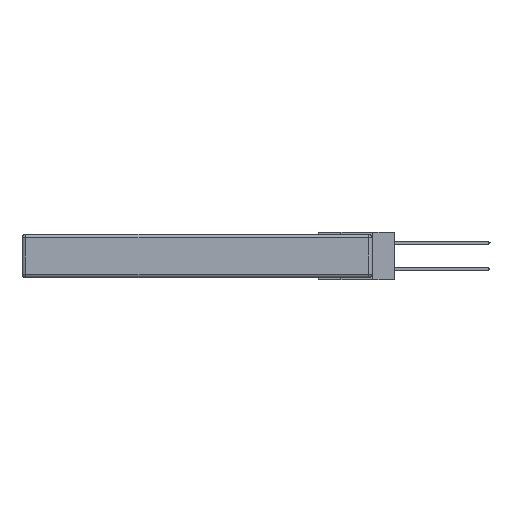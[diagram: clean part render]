
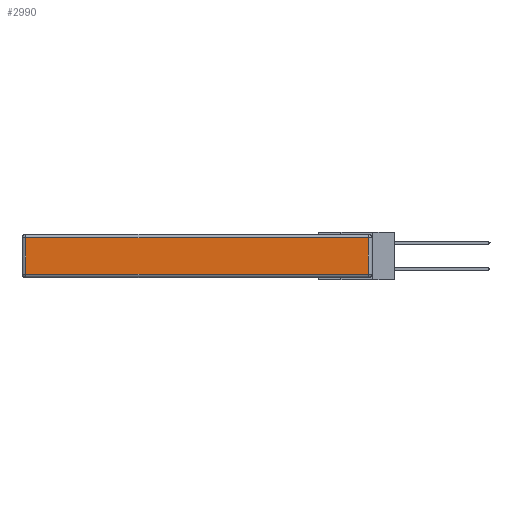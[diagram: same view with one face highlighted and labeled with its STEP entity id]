
A CAD part, left-side view. The second image highlights one B-rep face of the part: STEP entity #2990.
In plain terms, the highlighted planar face has unit normal (-1, 0, 0).
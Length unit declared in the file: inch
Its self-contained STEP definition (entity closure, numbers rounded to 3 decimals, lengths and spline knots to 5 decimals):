
#591 = DIRECTION ( 'NONE',  ( -1., 0., 0. ) ) ;
#1681 = DIRECTION ( 'NONE',  ( 0., -1., 0. ) ) ;
#1724 = CARTESIAN_POINT ( 'NONE',  ( 0., 2.72, -0.03 ) ) ;
#2984 = ORIENTED_EDGE ( 'NONE', *, *, #9275, .T. ) ;
#2990 = ADVANCED_FACE ( 'NONE', ( #14265 ), #3807, .T. ) ;
#3807 = PLANE ( 'NONE',  #13446 ) ;
#4156 = LINE ( 'NONE', #6775, #8483 ) ;
#4267 = DIRECTION ( 'NONE',  ( 0., 0., 1. ) ) ;
#5326 = CARTESIAN_POINT ( 'NONE',  ( 0., 0., -0.343 ) ) ;
#5942 = VECTOR ( 'NONE', #11424, 39.37008 ) ;
#6760 = CARTESIAN_POINT ( 'NONE',  ( 0., 2.72, -0.343 ) ) ;
#6775 = CARTESIAN_POINT ( 'NONE',  ( 0., 0., -0.313 ) ) ;
#7782 = VERTEX_POINT ( 'NONE', #13369 ) ;
#8369 = EDGE_LOOP ( 'NONE', ( #2984, #10035, #15524, #19790 ) ) ;
#8483 = VECTOR ( 'NONE', #1681, 39.37008 ) ;
#8833 = EDGE_CURVE ( 'NONE', #16061, #19935, #16183, .T. ) ;
#9275 = EDGE_CURVE ( 'NONE', #7782, #18838, #4156, .T. ) ;
#9654 = LINE ( 'NONE', #6760, #14544 ) ;
#9925 = CARTESIAN_POINT ( 'NONE',  ( 0., 2.75, -0.03 ) ) ;
#10035 = ORIENTED_EDGE ( 'NONE', *, *, #15393, .T. ) ;
#10290 = LINE ( 'NONE', #10875, #19941 ) ;
#10875 = CARTESIAN_POINT ( 'NONE',  ( 0., 0.03, -0.343 ) ) ;
#11424 = DIRECTION ( 'NONE',  ( 0., 1., 0. ) ) ;
#13369 = CARTESIAN_POINT ( 'NONE',  ( 0., 2.72, -0.313 ) ) ;
#13446 = AXIS2_PLACEMENT_3D ( 'NONE', #5326, #591, #18309 ) ;
#14265 = FACE_OUTER_BOUND ( 'NONE', #8369, .T. ) ;
#14544 = VECTOR ( 'NONE', #20107, 39.37008 ) ;
#15393 = EDGE_CURVE ( 'NONE', #18838, #16061, #10290, .T. ) ;
#15524 = ORIENTED_EDGE ( 'NONE', *, *, #8833, .T. ) ;
#16061 = VERTEX_POINT ( 'NONE', #20292 ) ;
#16183 = LINE ( 'NONE', #9925, #5942 ) ;
#18309 = DIRECTION ( 'NONE',  ( 0., 0., 1. ) ) ;
#18838 = VERTEX_POINT ( 'NONE', #19008 ) ;
#19008 = CARTESIAN_POINT ( 'NONE',  ( 0., 0.03, -0.313 ) ) ;
#19790 = ORIENTED_EDGE ( 'NONE', *, *, #20570, .T. ) ;
#19935 = VERTEX_POINT ( 'NONE', #1724 ) ;
#19941 = VECTOR ( 'NONE', #4267, 39.37008 ) ;
#20107 = DIRECTION ( 'NONE',  ( 0., 0., -1. ) ) ;
#20292 = CARTESIAN_POINT ( 'NONE',  ( 0., 0.03, -0.03 ) ) ;
#20570 = EDGE_CURVE ( 'NONE', #19935, #7782, #9654, .T. ) ;
